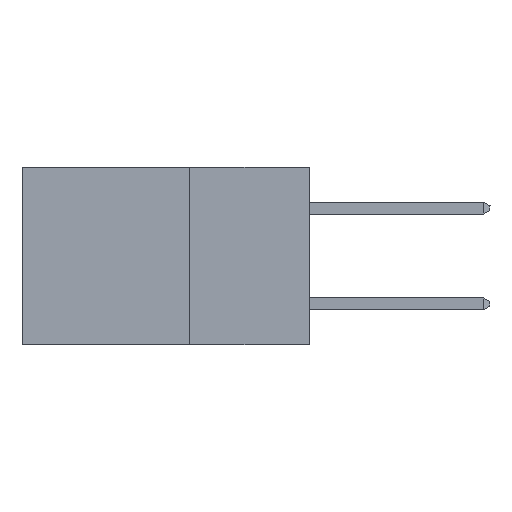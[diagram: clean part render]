
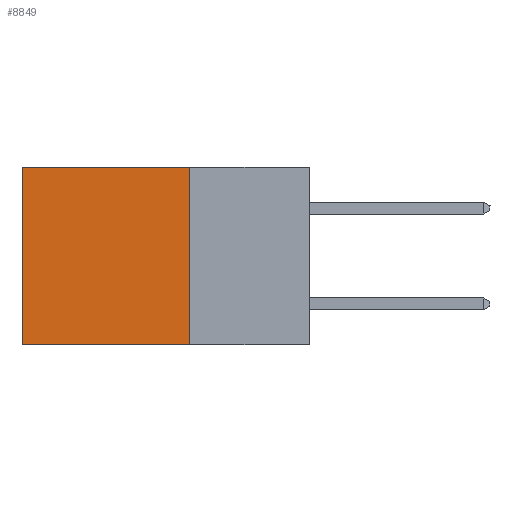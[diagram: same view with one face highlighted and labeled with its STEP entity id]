
A CAD part, left-side view. The second image highlights one B-rep face of the part: STEP entity #8849.
In plain terms, the highlighted planar face has unit normal (-1, 0, 0).
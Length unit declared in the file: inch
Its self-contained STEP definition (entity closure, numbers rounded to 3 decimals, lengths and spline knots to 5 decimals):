
#833 = DIRECTION ( 'NONE',  ( 0., 1., 0. ) ) ;
#1355 = CARTESIAN_POINT ( 'NONE',  ( 0.2875, 0.25, -0.37 ) ) ;
#2907 = DIRECTION ( 'NONE',  ( 0., 0., -1. ) ) ;
#3338 = ORIENTED_EDGE ( 'NONE', *, *, #4277, .F. ) ;
#3859 = CARTESIAN_POINT ( 'NONE',  ( 0.2875, 0.25, 0. ) ) ;
#4277 = EDGE_CURVE ( 'NONE', #8100, #9537, #10254, .T. ) ;
#4331 = VECTOR ( 'NONE', #11088, 39.37008 ) ;
#4575 = VECTOR ( 'NONE', #8240, 39.37008 ) ;
#4892 = LINE ( 'NONE', #6466, #4331 ) ;
#5164 = VERTEX_POINT ( 'NONE', #5392 ) ;
#5172 = CARTESIAN_POINT ( 'NONE',  ( 0.2875, 0.6, 0. ) ) ;
#5392 = CARTESIAN_POINT ( 'NONE',  ( 0.2875, 0.6, -0.37 ) ) ;
#5433 = VECTOR ( 'NONE', #2907, 39.37008 ) ;
#6023 = VERTEX_POINT ( 'NONE', #5172 ) ;
#6394 = DIRECTION ( 'NONE',  ( 0., 0., -1. ) ) ;
#6466 = CARTESIAN_POINT ( 'NONE',  ( 0.2875, 0.6, 0. ) ) ;
#6908 = EDGE_CURVE ( 'NONE', #9537, #5164, #7529, .T. ) ;
#7281 = CARTESIAN_POINT ( 'NONE',  ( 0.2875, 0.25, 0. ) ) ;
#7395 = ORIENTED_EDGE ( 'NONE', *, *, #9378, .T. ) ;
#7445 = CARTESIAN_POINT ( 'NONE',  ( 0.2875, 0.25, 0. ) ) ;
#7529 = LINE ( 'NONE', #9703, #9334 ) ;
#7571 = LINE ( 'NONE', #3859, #4575 ) ;
#7896 = FACE_OUTER_BOUND ( 'NONE', #11107, .T. ) ;
#8052 = ORIENTED_EDGE ( 'NONE', *, *, #6908, .F. ) ;
#8100 = VERTEX_POINT ( 'NONE', #8663 ) ;
#8116 = AXIS2_PLACEMENT_3D ( 'NONE', #7281, #9043, #6394 ) ;
#8240 = DIRECTION ( 'NONE',  ( 0., 1., 0. ) ) ;
#8663 = CARTESIAN_POINT ( 'NONE',  ( 0.2875, 0.25, 0. ) ) ;
#8772 = ORIENTED_EDGE ( 'NONE', *, *, #11295, .T. ) ;
#8849 = ADVANCED_FACE ( 'NONE', ( #7896 ), #9014, .F. ) ;
#9014 = PLANE ( 'NONE',  #8116 ) ;
#9043 = DIRECTION ( 'NONE',  ( 1., 0., 0. ) ) ;
#9334 = VECTOR ( 'NONE', #833, 39.37008 ) ;
#9378 = EDGE_CURVE ( 'NONE', #6023, #5164, #4892, .T. ) ;
#9537 = VERTEX_POINT ( 'NONE', #1355 ) ;
#9703 = CARTESIAN_POINT ( 'NONE',  ( 0.2875, 0.25, -0.37 ) ) ;
#10254 = LINE ( 'NONE', #7445, #5433 ) ;
#11088 = DIRECTION ( 'NONE',  ( 0., 0., -1. ) ) ;
#11107 = EDGE_LOOP ( 'NONE', ( #7395, #8052, #3338, #8772 ) ) ;
#11295 = EDGE_CURVE ( 'NONE', #8100, #6023, #7571, .T. ) ;
